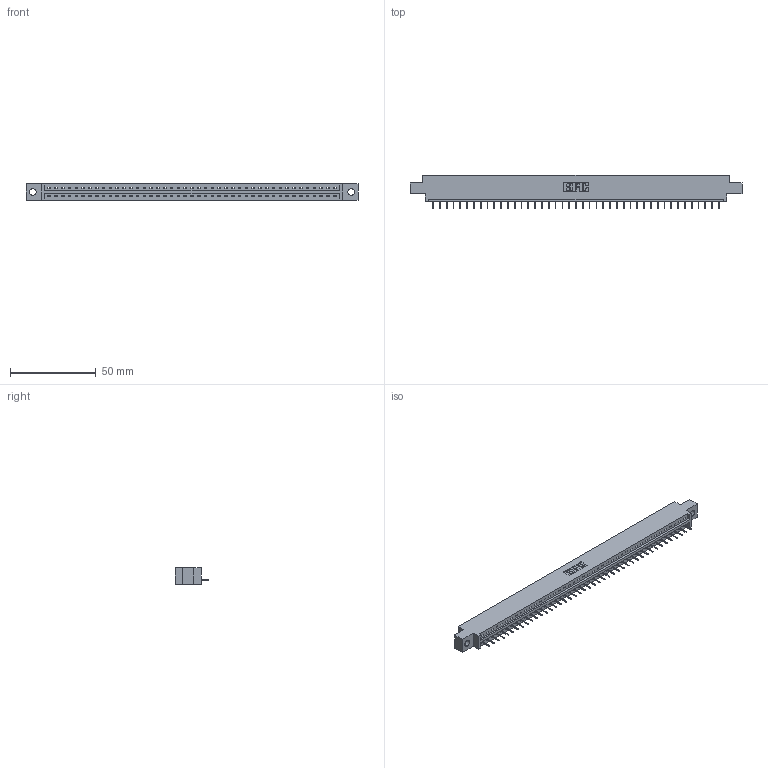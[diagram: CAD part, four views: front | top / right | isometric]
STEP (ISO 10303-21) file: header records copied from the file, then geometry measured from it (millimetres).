
FILE_DESCRIPTION (( 'STEP AP203' ), '1' );
FILE_NAME ('337-043-524-604.STEP', '2019-10-01T23:28:27', ( '' ), ( '' ), 'SwSTEP 2.0', 'SolidWorks 2016', '' );
FILE_SCHEMA (( 'CONFIG_CONTROL_DESIGN' ));
Length unit declared in the file: inch
Products named in the file (3): 337 Part_0.170 Offset - 0.156 Dia-TH; 337-043-524-604; 345-292-001_345-293-124
Assembly tree (44 placements, depth 2):
  337-043-524-604
    337 Part_0.170 Offset - 0.156 Dia-TH
    345-292-001_345-293-124  x43
Bounding box: 193.4 x 19.69 x 9.4 mm (x, y, z)
Volume: 19737.5 mm3; surface area: 19695.7 mm2
Topology: 44 solids, 44 shells, 2956 faces, 8579 edges, 5546 vertices
Faces by surface type: plane 2310, cylinder 646
Entity records: 32043 total; most frequent: CARTESIAN_POINT 5587, ORIENTED_EDGE 5566, DIRECTION 4701, EDGE_CURVE 2783, LINE 2659, VECTOR 2659, VERTEX_POINT 1850, AXIS2_PLACEMENT_3D 1021
